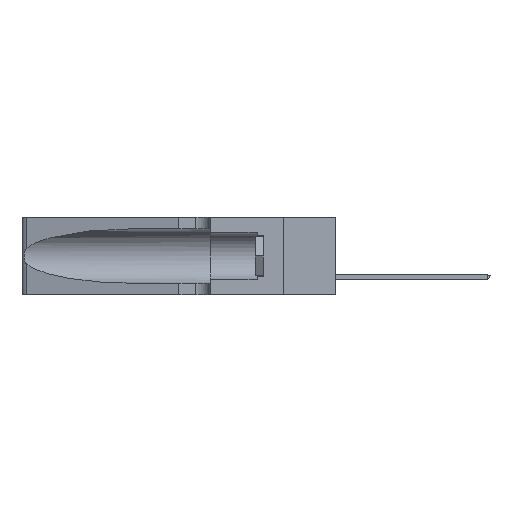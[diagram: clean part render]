
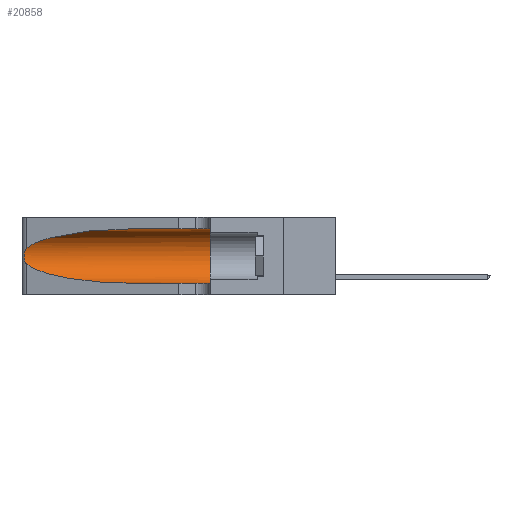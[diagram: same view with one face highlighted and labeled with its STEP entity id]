
A CAD part, left-side view. The second image highlights one B-rep face of the part: STEP entity #20858.
In plain terms, the highlighted cylindrical face has radius 3.308 mm (diameter 6.617 mm), a partial arc.
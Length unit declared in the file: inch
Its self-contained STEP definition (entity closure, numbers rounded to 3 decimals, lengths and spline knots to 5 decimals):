
#109 = CARTESIAN_POINT ( 'NONE',  ( 0.26075, 1.23896, 0.178 ) ) ;
#808 = VERTEX_POINT ( 'NONE', #26119 ) ;
#820 = CARTESIAN_POINT ( 'NONE',  ( 0.2373, 1.15595, 0.08982 ) ) ;
#1908 = CARTESIAN_POINT ( 'NONE',  ( 0.1305, 1.61858, 0.31525 ) ) ;
#1924 = ORIENTED_EDGE ( 'NONE', *, *, #18755, .T. ) ;
#2819 = VERTEX_POINT ( 'NONE', #8556 ) ;
#2845 = DIRECTION ( 'NONE',  ( 0., -1., 0. ) ) ;
#3665 = ORIENTED_EDGE ( 'NONE', *, *, #31175, .T. ) ;
#4567 = VERTEX_POINT ( 'NONE', #6937 ) ;
#5365 = DIRECTION ( 'NONE',  ( 0., -1., 0. ) ) ;
#5835 = CIRCLE ( 'NONE', #21614, 0.13025 ) ;
#6937 = CARTESIAN_POINT ( 'NONE',  ( 0.25487, 1.22718, 0.22369 ) ) ;
#7077 = CARTESIAN_POINT ( 'NONE',  ( 0.1305, 0.35, 0.185 ) ) ;
#7434 = CARTESIAN_POINT ( 'NONE',  ( 0.1305, 1.61858, 0.185 ) ) ;
#7524 = B_SPLINE_CURVE_WITH_KNOTS ( 'NONE', 3,
 ( #25097, #13492, #28643, #12267, #8974, #29810, #39083, #109, #35882, #11750, #17857, #18217, #36017, #24147 ),
 .UNSPECIFIED., .F., .F.,
 ( 4, 2, 2, 2, 2, 2, 4 ),
 ( 0., 0.00027, 0.00053, 0.00107, 0.0016, 0.00187, 0.00214 ),
 .UNSPECIFIED. ) ;
#7721 = ORIENTED_EDGE ( 'NONE', *, *, #27794, .F. ) ;
#8556 = CARTESIAN_POINT ( 'NONE',  ( 0.1305, 0.72297, 0.31525 ) ) ;
#8974 = CARTESIAN_POINT ( 'NONE',  ( 0.25854, 1.2359, 0.20912 ) ) ;
#9031 = CARTESIAN_POINT ( 'NONE',  ( 0.1305, 0.35, 0.05475 ) ) ;
#11320 = CARTESIAN_POINT ( 'NONE',  ( 0.2373, 1.15595, 0.28018 ) ) ;
#11566 = AXIS2_PLACEMENT_3D ( 'NONE', #7434, #13498, #16282 ) ;
#11593 = CARTESIAN_POINT ( 'NONE',  ( 0.18966, 0.96281, 0.31525 ) ) ;
#11750 = CARTESIAN_POINT ( 'NONE',  ( 0.25856, 1.23593, 0.16098 ) ) ;
#12086 = CARTESIAN_POINT ( 'NONE',  ( 0.1305, 1.61858, 0.05475 ) ) ;
#12263 = EDGE_CURVE ( 'NONE', #2819, #4567, #36768, .T. ) ;
#12267 = CARTESIAN_POINT ( 'NONE',  ( 0.25787, 1.23484, 0.2124 ) ) ;
#12726 = EDGE_CURVE ( 'NONE', #2819, #38546, #24582, .T. ) ;
#13492 = CARTESIAN_POINT ( 'NONE',  ( 0.25555, 1.22994, 0.2215 ) ) ;
#13498 = DIRECTION ( 'NONE',  ( 0., -1., 0. ) ) ;
#14614 = CARTESIAN_POINT ( 'NONE',  ( 0.1305, 0.72297, 0.05475 ) ) ;
#16202 = DIRECTION ( 'NONE',  ( 0., 0., 1. ) ) ;
#16282 = DIRECTION ( 'NONE',  ( 0., 0., -1. ) ) ;
#17857 = CARTESIAN_POINT ( 'NONE',  ( 0.25789, 1.23486, 0.15765 ) ) ;
#18217 = CARTESIAN_POINT ( 'NONE',  ( 0.25639, 1.23186, 0.15144 ) ) ;
#18575 = VECTOR ( 'NONE', #2845, 39.37008 ) ;
#18755 = EDGE_CURVE ( 'NONE', #4567, #808, #7524, .T. ) ;
#19741 = ORIENTED_EDGE ( 'NONE', *, *, #32912, .T. ) ;
#20028 = CARTESIAN_POINT ( 'NONE',  ( 0.1305, 0.35, 0.31525 ) ) ;
#20741 = CARTESIAN_POINT ( 'NONE',  ( 0.1305, 0.72297, 0.31525 ) ) ;
#20858 = ADVANCED_FACE ( 'NONE', ( #39041 ), #25803, .F. ) ;
#21550 = VERTEX_POINT ( 'NONE', #14614 ) ;
#21614 = AXIS2_PLACEMENT_3D ( 'NONE', #7077, #25030, #16202 ) ;
#22388 = EDGE_LOOP ( 'NONE', ( #28742, #1924, #3665, #19741, #7721, #29851 ) ) ;
#22941 = VERTEX_POINT ( 'NONE', #9031 ) ;
#24147 = CARTESIAN_POINT ( 'NONE',  ( 0.25487, 1.22718, 0.14631 ) ) ;
#24582 = LINE ( 'NONE', #1908, #38296 ) ;
#25005 = CARTESIAN_POINT ( 'NONE',  ( 0.25487, 1.22718, 0.14631 ) ) ;
#25030 = DIRECTION ( 'NONE',  ( 0., 1., 0. ) ) ;
#25097 = CARTESIAN_POINT ( 'NONE',  ( 0.25487, 1.22718, 0.22369 ) ) ;
#25803 = CYLINDRICAL_SURFACE ( 'NONE', #11566, 0.13025 ) ;
#26091 = LINE ( 'NONE', #12086, #18575 ) ;
#26119 = CARTESIAN_POINT ( 'NONE',  ( 0.25487, 1.22718, 0.14631 ) ) ;
#27794 = EDGE_CURVE ( 'NONE', #38546, #22941, #5835, .T. ) ;
#28643 = CARTESIAN_POINT ( 'NONE',  ( 0.25639, 1.23184, 0.21858 ) ) ;
#28742 = ORIENTED_EDGE ( 'NONE', *, *, #12263, .T. ) ;
#29785 = CARTESIAN_POINT ( 'NONE',  ( 0.25487, 1.22718, 0.22369 ) ) ;
#29810 = CARTESIAN_POINT ( 'NONE',  ( 0.26018, 1.23835, 0.19895 ) ) ;
#29851 = ORIENTED_EDGE ( 'NONE', *, *, #12726, .F. ) ;
#30741 =( BOUNDED_CURVE ( )  B_SPLINE_CURVE ( 3, ( #25005, #820, #30796, #34232 ),
 .UNSPECIFIED., .F., .T. ) 
 B_SPLINE_CURVE_WITH_KNOTS ( ( 4, 4 ),
 ( 3.44316, 4.71239 ),
 .UNSPECIFIED. ) 
 CURVE ( )  GEOMETRIC_REPRESENTATION_ITEM ( )  RATIONAL_B_SPLINE_CURVE ( ( 1., 0.87, 0.87, 1. ) ) 
 REPRESENTATION_ITEM ( '' )  );
#30796 = CARTESIAN_POINT ( 'NONE',  ( 0.18966, 0.96281, 0.05475 ) ) ;
#31175 = EDGE_CURVE ( 'NONE', #808, #21550, #30741, .T. ) ;
#32912 = EDGE_CURVE ( 'NONE', #21550, #22941, #26091, .T. ) ;
#34232 = CARTESIAN_POINT ( 'NONE',  ( 0.1305, 0.72297, 0.05475 ) ) ;
#35882 = CARTESIAN_POINT ( 'NONE',  ( 0.26017, 1.23833, 0.17102 ) ) ;
#36017 = CARTESIAN_POINT ( 'NONE',  ( 0.25555, 1.22993, 0.14849 ) ) ;
#36768 =( BOUNDED_CURVE ( )  B_SPLINE_CURVE ( 3, ( #20741, #11593, #11320, #29785 ),
 .UNSPECIFIED., .F., .T. ) 
 B_SPLINE_CURVE_WITH_KNOTS ( ( 4, 4 ),
 ( 1.5708, 2.84003 ),
 .UNSPECIFIED. ) 
 CURVE ( )  GEOMETRIC_REPRESENTATION_ITEM ( )  RATIONAL_B_SPLINE_CURVE ( ( 1., 0.87, 0.87, 1. ) ) 
 REPRESENTATION_ITEM ( '' )  );
#38296 = VECTOR ( 'NONE', #5365, 39.37008 ) ;
#38546 = VERTEX_POINT ( 'NONE', #20028 ) ;
#39041 = FACE_OUTER_BOUND ( 'NONE', #22388, .T. ) ;
#39083 = CARTESIAN_POINT ( 'NONE',  ( 0.26075, 1.23896, 0.19203 ) ) ;
